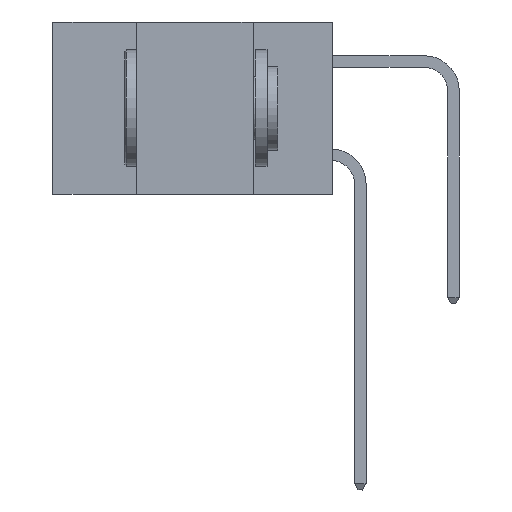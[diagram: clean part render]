
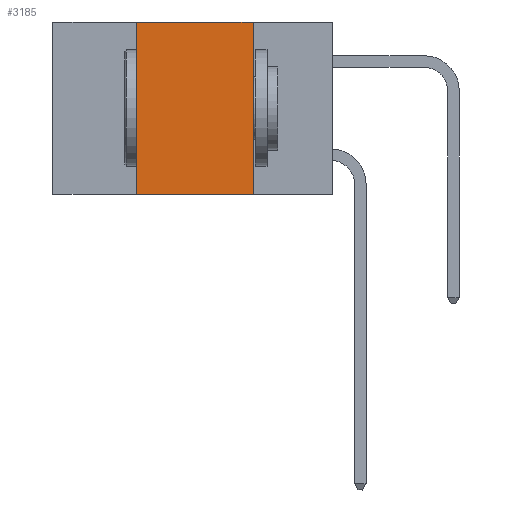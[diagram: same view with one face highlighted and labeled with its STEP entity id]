
A CAD part, left-side view. The second image highlights one B-rep face of the part: STEP entity #3185.
In plain terms, the highlighted planar face has unit normal (-1, 0, 0).
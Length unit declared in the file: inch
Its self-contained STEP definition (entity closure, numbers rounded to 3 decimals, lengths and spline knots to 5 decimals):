
#107 = CARTESIAN_POINT ( 'NONE',  ( 0., 0.42, 0. ) ) ;
#286 = DIRECTION ( 'NONE',  ( 1., 0., 0. ) ) ;
#503 = CARTESIAN_POINT ( 'NONE',  ( 0., 0.17, -0.37 ) ) ;
#541 = PLANE ( 'NONE',  #10300 ) ;
#1243 = VECTOR ( 'NONE', #9817, 39.37008 ) ;
#1465 = CARTESIAN_POINT ( 'NONE',  ( 0., 0.6, 0. ) ) ;
#1840 = CARTESIAN_POINT ( 'NONE',  ( 0., 0.17, 0. ) ) ;
#2041 = ORIENTED_EDGE ( 'NONE', *, *, #9017, .F. ) ;
#2311 = ORIENTED_EDGE ( 'NONE', *, *, #7620, .T. ) ;
#2713 = VECTOR ( 'NONE', #12318, 39.37008 ) ;
#3102 = DIRECTION ( 'NONE',  ( 0., 0., 1. ) ) ;
#3171 = VECTOR ( 'NONE', #6677, 39.37008 ) ;
#3185 = ADVANCED_FACE ( 'NONE', ( #4181 ), #541, .F. ) ;
#3228 = EDGE_CURVE ( 'NONE', #12233, #9664, #3875, .T. ) ;
#3535 = DIRECTION ( 'NONE',  ( 0., 0., -1. ) ) ;
#3875 = LINE ( 'NONE', #1465, #1243 ) ;
#4181 = FACE_OUTER_BOUND ( 'NONE', #5385, .T. ) ;
#4342 = ORIENTED_EDGE ( 'NONE', *, *, #3228, .F. ) ;
#4625 = CARTESIAN_POINT ( 'NONE',  ( 0., 0.17, 0. ) ) ;
#5385 = EDGE_LOOP ( 'NONE', ( #11016, #4342, #2041, #2311 ) ) ;
#5444 = LINE ( 'NONE', #107, #7712 ) ;
#6044 = LINE ( 'NONE', #12425, #3171 ) ;
#6489 = VERTEX_POINT ( 'NONE', #10829 ) ;
#6677 = DIRECTION ( 'NONE',  ( 0., -1., 0. ) ) ;
#7620 = EDGE_CURVE ( 'NONE', #6489, #8636, #6044, .T. ) ;
#7712 = VECTOR ( 'NONE', #3102, 39.37008 ) ;
#7839 = CARTESIAN_POINT ( 'NONE',  ( 0., 0.6, 0. ) ) ;
#8029 = CARTESIAN_POINT ( 'NONE',  ( 0., 0.42, 0. ) ) ;
#8636 = VERTEX_POINT ( 'NONE', #503 ) ;
#8761 = EDGE_CURVE ( 'NONE', #9664, #8636, #10455, .T. ) ;
#9017 = EDGE_CURVE ( 'NONE', #6489, #12233, #5444, .T. ) ;
#9664 = VERTEX_POINT ( 'NONE', #1840 ) ;
#9817 = DIRECTION ( 'NONE',  ( 0., -1., 0. ) ) ;
#10300 = AXIS2_PLACEMENT_3D ( 'NONE', #7839, #286, #3535 ) ;
#10455 = LINE ( 'NONE', #4625, #2713 ) ;
#10829 = CARTESIAN_POINT ( 'NONE',  ( 0., 0.42, -0.37 ) ) ;
#11016 = ORIENTED_EDGE ( 'NONE', *, *, #8761, .F. ) ;
#12233 = VERTEX_POINT ( 'NONE', #8029 ) ;
#12318 = DIRECTION ( 'NONE',  ( 0., 0., -1. ) ) ;
#12425 = CARTESIAN_POINT ( 'NONE',  ( 0., 0.6, -0.37 ) ) ;
